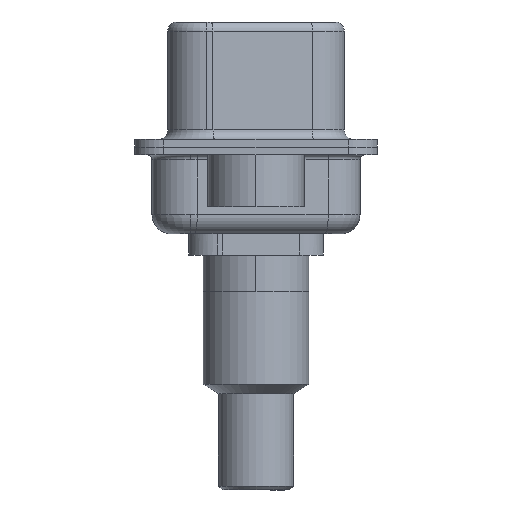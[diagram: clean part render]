
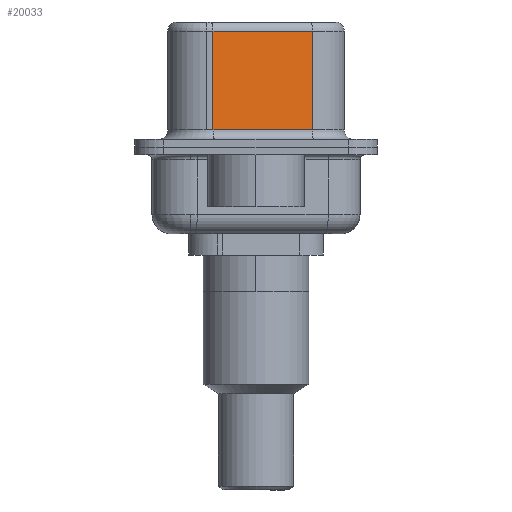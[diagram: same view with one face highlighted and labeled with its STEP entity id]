
A CAD part, left-side view. The second image highlights one B-rep face of the part: STEP entity #20033.
In plain terms, the highlighted planar face has unit normal (-0.985, -0.174, 0).
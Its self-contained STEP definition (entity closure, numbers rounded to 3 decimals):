
#251 = CARTESIAN_POINT ( 'NONE',  ( 4.585, -2.927, 6.02 ) ) ;
#581 = EDGE_CURVE ( 'NONE', #12942, #16986, #4122, .T. ) ;
#622 = EDGE_CURVE ( 'NONE', #3187, #16986, #3558, .T. ) ;
#1508 = ORIENTED_EDGE ( 'NONE', *, *, #1759, .T. ) ;
#1759 = EDGE_CURVE ( 'NONE', #3187, #3934, #15768, .T. ) ;
#2515 = VECTOR ( 'NONE', #16034, 1000. ) ;
#3187 = VERTEX_POINT ( 'NONE', #251 ) ;
#3558 = LINE ( 'NONE', #10959, #12777 ) ;
#3934 = VERTEX_POINT ( 'NONE', #19835 ) ;
#4122 = LINE ( 'NONE', #8928, #13316 ) ;
#4302 = DIRECTION ( 'NONE',  ( -0.174, 0.985, 0. ) ) ;
#5030 = DIRECTION ( 'NONE',  ( -0.174, 0.985, 0. ) ) ;
#5264 = DIRECTION ( 'NONE',  ( 0., 0., -1. ) ) ;
#6015 = VECTOR ( 'NONE', #4302, 1000. ) ;
#6801 = EDGE_CURVE ( 'NONE', #3934, #12942, #7335, .T. ) ;
#7335 = LINE ( 'NONE', #14231, #2515 ) ;
#8928 = CARTESIAN_POINT ( 'NONE',  ( 4.585, -2.927, 0.9 ) ) ;
#9162 = CARTESIAN_POINT ( 'NONE',  ( 3.675, 2.233, 0.9 ) ) ;
#9583 = AXIS2_PLACEMENT_3D ( 'NONE', #17732, #15990, #5030 ) ;
#10160 = FACE_OUTER_BOUND ( 'NONE', #13563, .T. ) ;
#10959 = CARTESIAN_POINT ( 'NONE',  ( 4.585, -2.927, 6.52 ) ) ;
#12777 = VECTOR ( 'NONE', #5264, 1000. ) ;
#12942 = VERTEX_POINT ( 'NONE', #9162 ) ;
#13316 = VECTOR ( 'NONE', #16828, 1000. ) ;
#13391 = CARTESIAN_POINT ( 'NONE',  ( 4.585, -2.927, 6.02 ) ) ;
#13563 = EDGE_LOOP ( 'NONE', ( #16604, #1508, #20270, #20765 ) ) ;
#14190 = PLANE ( 'NONE',  #9583 ) ;
#14231 = CARTESIAN_POINT ( 'NONE',  ( 3.675, 2.233, 6.52 ) ) ;
#15768 = LINE ( 'NONE', #13391, #6015 ) ;
#15990 = DIRECTION ( 'NONE',  ( 0.985, 0.174, 0. ) ) ;
#16034 = DIRECTION ( 'NONE',  ( 0., 0., -1. ) ) ;
#16604 = ORIENTED_EDGE ( 'NONE', *, *, #622, .F. ) ;
#16828 = DIRECTION ( 'NONE',  ( 0.174, -0.985, 0. ) ) ;
#16986 = VERTEX_POINT ( 'NONE', #19965 ) ;
#17732 = CARTESIAN_POINT ( 'NONE',  ( 4.585, -2.927, 6.52 ) ) ;
#19835 = CARTESIAN_POINT ( 'NONE',  ( 3.675, 2.233, 6.02 ) ) ;
#19965 = CARTESIAN_POINT ( 'NONE',  ( 4.585, -2.927, 0.9 ) ) ;
#20033 = ADVANCED_FACE ( 'NONE', ( #10160 ), #14190, .F. ) ;
#20270 = ORIENTED_EDGE ( 'NONE', *, *, #6801, .T. ) ;
#20765 = ORIENTED_EDGE ( 'NONE', *, *, #581, .T. ) ;
